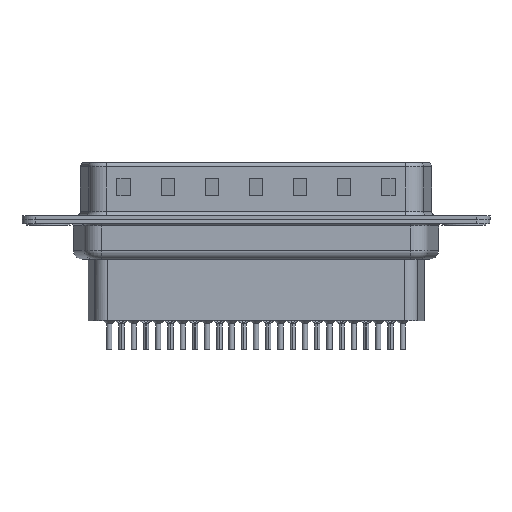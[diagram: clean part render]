
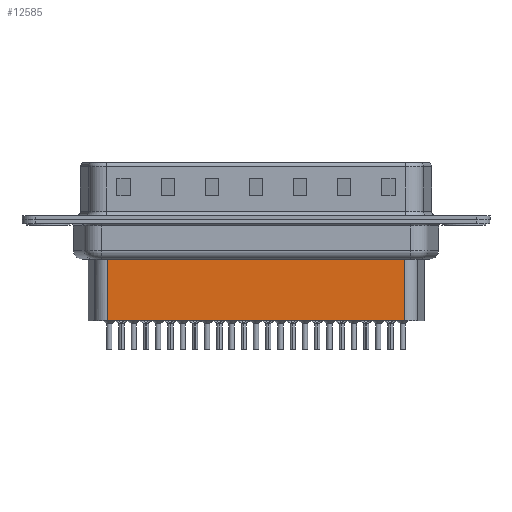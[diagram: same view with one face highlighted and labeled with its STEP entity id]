
A CAD part, front view. The second image highlights one B-rep face of the part: STEP entity #12585.
In plain terms, the highlighted planar face has unit normal (0, -1, 0).
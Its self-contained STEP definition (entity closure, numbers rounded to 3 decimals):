
#552 = VERTEX_POINT ( 'NONE', #20654 ) ;
#1952 = EDGE_CURVE ( 'NONE', #6297, #11612, #22049, .T. ) ;
#2466 = DIRECTION ( 'NONE',  ( -1., 0., 0. ) ) ;
#2543 = LINE ( 'NONE', #2729, #21117 ) ;
#2729 = CARTESIAN_POINT ( 'NONE',  ( 40.344, -3.5, -3.1 ) ) ;
#3128 = EDGE_CURVE ( 'NONE', #12986, #6297, #18018, .T. ) ;
#4965 = EDGE_CURVE ( 'NONE', #12986, #552, #2543, .T. ) ;
#5358 = DIRECTION ( 'NONE',  ( 0., -1., 0. ) ) ;
#6297 = VERTEX_POINT ( 'NONE', #19860 ) ;
#6996 = DIRECTION ( 'NONE',  ( 0., 0., -1. ) ) ;
#7609 = CARTESIAN_POINT ( 'NONE',  ( 6.706, -3.5, -11.45 ) ) ;
#7722 = CARTESIAN_POINT ( 'NONE',  ( 6.459, -3.5, -4.097 ) ) ;
#8485 = VECTOR ( 'NONE', #2466, 1000. ) ;
#10037 = CARTESIAN_POINT ( 'NONE',  ( 40.344, -3.5, -4.097 ) ) ;
#11505 = CARTESIAN_POINT ( 'NONE',  ( 6.706, -3.5, -11.45 ) ) ;
#11612 = VERTEX_POINT ( 'NONE', #11505 ) ;
#11705 = AXIS2_PLACEMENT_3D ( 'NONE', #16096, #5358, #17889 ) ;
#11897 = ORIENTED_EDGE ( 'NONE', *, *, #14148, .F. ) ;
#12117 = ORIENTED_EDGE ( 'NONE', *, *, #4965, .F. ) ;
#12585 = ADVANCED_FACE ( 'NONE', ( #20677 ), #23302, .T. ) ;
#12986 = VERTEX_POINT ( 'NONE', #10037 ) ;
#13282 = ORIENTED_EDGE ( 'NONE', *, *, #1952, .T. ) ;
#14148 = EDGE_CURVE ( 'NONE', #552, #11612, #15805, .T. ) ;
#15805 = LINE ( 'NONE', #7609, #20040 ) ;
#16096 = CARTESIAN_POINT ( 'NONE',  ( 6.706, -3.5, -3.1 ) ) ;
#17219 = VECTOR ( 'NONE', #6996, 1000. ) ;
#17348 = CARTESIAN_POINT ( 'NONE',  ( 6.706, -3.5, -3.1 ) ) ;
#17889 = DIRECTION ( 'NONE',  ( 1., 0., 0. ) ) ;
#18018 = LINE ( 'NONE', #7722, #8485 ) ;
#19860 = CARTESIAN_POINT ( 'NONE',  ( 6.706, -3.5, -4.097 ) ) ;
#20040 = VECTOR ( 'NONE', #20200, 1000. ) ;
#20200 = DIRECTION ( 'NONE',  ( -1., 0., 0. ) ) ;
#20654 = CARTESIAN_POINT ( 'NONE',  ( 40.344, -3.5, -11.45 ) ) ;
#20677 = FACE_OUTER_BOUND ( 'NONE', #21138, .T. ) ;
#20758 = ORIENTED_EDGE ( 'NONE', *, *, #3128, .T. ) ;
#21117 = VECTOR ( 'NONE', #21266, 1000. ) ;
#21138 = EDGE_LOOP ( 'NONE', ( #12117, #20758, #13282, #11897 ) ) ;
#21266 = DIRECTION ( 'NONE',  ( 0., 0., -1. ) ) ;
#22049 = LINE ( 'NONE', #17348, #17219 ) ;
#23302 = PLANE ( 'NONE',  #11705 ) ;
